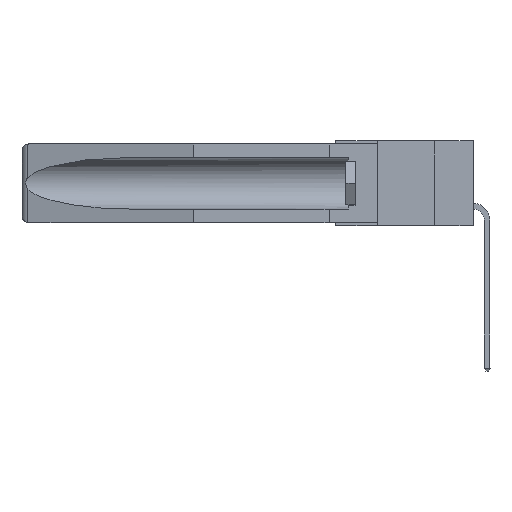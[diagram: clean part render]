
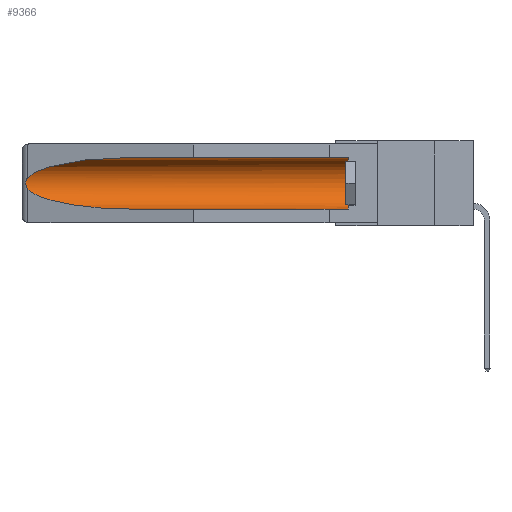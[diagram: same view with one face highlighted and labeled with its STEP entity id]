
A CAD part, left-side view. The second image highlights one B-rep face of the part: STEP entity #9366.
In plain terms, the highlighted cylindrical face has radius 2.857 mm (diameter 5.715 mm), a partial arc.
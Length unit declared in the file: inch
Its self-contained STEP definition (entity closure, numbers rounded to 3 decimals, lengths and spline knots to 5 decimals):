
#129 = CARTESIAN_POINT ( 'NONE',  ( 0.26654, 1.53092, -0.15636 ) ) ;
#334 = CARTESIAN_POINT ( 'NONE',  ( 0.21114, 1.30732, -0.284 ) ) ;
#395 = LINE ( 'NONE', #983, #7220 ) ;
#399 = CARTESIAN_POINT ( 'NONE',  ( 0.155, 0.126, -0.059 ) ) ;
#403 = ORIENTED_EDGE ( 'NONE', *, *, #19770, .T. ) ;
#882 = EDGE_CURVE ( 'NONE', #8892, #11822, #16762, .T. ) ;
#983 = CARTESIAN_POINT ( 'NONE',  ( 0.155, -0.30754, -0.059 ) ) ;
#1726 = EDGE_CURVE ( 'NONE', #2985, #11822, #15769, .T. ) ;
#1744 = CARTESIAN_POINT ( 'NONE',  ( 0.2673, 1.53269, -0.17917 ) ) ;
#1752 = CARTESIAN_POINT ( 'NONE',  ( 0.25451, 1.48313, -0.09465 ) ) ;
#2117 = CARTESIAN_POINT ( 'NONE',  ( 0.26537, 1.52718, -0.19328 ) ) ;
#2985 = VERTEX_POINT ( 'NONE', #2117 ) ;
#3013 = ORIENTED_EDGE ( 'NONE', *, *, #8179, .T. ) ;
#3300 = AXIS2_PLACEMENT_3D ( 'NONE', #17911, #8247, #13104 ) ;
#3367 = CARTESIAN_POINT ( 'NONE',  ( 0.26537, 1.52718, -0.19328 ) ) ;
#3433 = CARTESIAN_POINT ( 'NONE',  ( 0.25451, 1.48313, -0.24835 ) ) ;
#3542 = VERTEX_POINT ( 'NONE', #399 ) ;
#4724 = CYLINDRICAL_SURFACE ( 'NONE', #6456, 0.1125 ) ;
#4879 = CARTESIAN_POINT ( 'NONE',  ( 0.26597, 1.5296, -0.19026 ) ) ;
#5089 = CARTESIAN_POINT ( 'NONE',  ( 0.155, 1.07973, -0.284 ) ) ;
#6266 = DIRECTION ( 'NONE',  ( 0., 1., 0. ) ) ;
#6456 = AXIS2_PLACEMENT_3D ( 'NONE', #15570, #17184, #18846 ) ;
#6930 = CARTESIAN_POINT ( 'NONE',  ( 0.155, 0.126, -0.284 ) ) ;
#7220 = VECTOR ( 'NONE', #8891, 39.37008 ) ;
#8179 = EDGE_CURVE ( 'NONE', #18957, #16671, #12662, .T. ) ;
#8247 = DIRECTION ( 'NONE',  ( 0., -1., 0. ) ) ;
#8891 = DIRECTION ( 'NONE',  ( 0., 1., 0. ) ) ;
#8892 = VERTEX_POINT ( 'NONE', #6930 ) ;
#9040 = CARTESIAN_POINT ( 'NONE',  ( 0.155, 1.07973, -0.059 ) ) ;
#9366 = ADVANCED_FACE ( 'NONE', ( #10301 ), #4724, .F. ) ;
#9506 = CARTESIAN_POINT ( 'NONE',  ( 0.26537, 1.52718, -0.14972 ) ) ;
#9737 = CARTESIAN_POINT ( 'NONE',  ( 0.155, 1.07973, -0.059 ) ) ;
#9948 = CARTESIAN_POINT ( 'NONE',  ( 0.2675, 1.53308, -0.17534 ) ) ;
#10095 = CARTESIAN_POINT ( 'NONE',  ( 0.26537, 1.52718, -0.14972 ) ) ;
#10301 = FACE_OUTER_BOUND ( 'NONE', #13452, .T. ) ;
#11099 = B_SPLINE_CURVE_WITH_KNOTS ( 'NONE', 3,
 ( #13170, #17970, #129, #14580, #14729, #9948, #1744, #13092, #4879, #16189 ),
 .UNSPECIFIED., .F., .F.,
 ( 4, 2, 2, 2, 4 ),
 ( 0., 0.00029, 0.00058, 0.00087, 0.00117 ),
 .UNSPECIFIED. ) ;
#11822 = VERTEX_POINT ( 'NONE', #19380 ) ;
#11911 = ORIENTED_EDGE ( 'NONE', *, *, #18937, .T. ) ;
#12368 = CIRCLE ( 'NONE', #3300, 0.1125 ) ;
#12662 =( BOUNDED_CURVE ( )  B_SPLINE_CURVE ( 3, ( #9737, #12726, #1752, #10095 ),
 .UNSPECIFIED., .F., .F. ) 
 B_SPLINE_CURVE_WITH_KNOTS ( ( 4, 4 ),
 ( 4.71239, 6.08839 ),
 .UNSPECIFIED. ) 
 CURVE ( )  GEOMETRIC_REPRESENTATION_ITEM ( )  RATIONAL_B_SPLINE_CURVE ( ( 1., 0.848, 0.848, 1. ) ) 
 REPRESENTATION_ITEM ( '' )  );
#12726 = CARTESIAN_POINT ( 'NONE',  ( 0.21114, 1.30732, -0.059 ) ) ;
#13092 = CARTESIAN_POINT ( 'NONE',  ( 0.26655, 1.53094, -0.18657 ) ) ;
#13104 = DIRECTION ( 'NONE',  ( 0., 0., 1. ) ) ;
#13170 = CARTESIAN_POINT ( 'NONE',  ( 0.26537, 1.52718, -0.14972 ) ) ;
#13452 = EDGE_LOOP ( 'NONE', ( #3013, #403, #13462, #18812, #20100, #11911 ) ) ;
#13462 = ORIENTED_EDGE ( 'NONE', *, *, #1726, .T. ) ;
#14580 = CARTESIAN_POINT ( 'NONE',  ( 0.2673, 1.5327, -0.16383 ) ) ;
#14729 = CARTESIAN_POINT ( 'NONE',  ( 0.2675, 1.53308, -0.16763 ) ) ;
#15543 = EDGE_CURVE ( 'NONE', #8892, #3542, #12368, .T. ) ;
#15570 = CARTESIAN_POINT ( 'NONE',  ( 0.155, -0.30754, -0.1715 ) ) ;
#15769 =( BOUNDED_CURVE ( )  B_SPLINE_CURVE ( 3, ( #3367, #3433, #334, #5089 ),
 .UNSPECIFIED., .F., .T. ) 
 B_SPLINE_CURVE_WITH_KNOTS ( ( 4, 4 ),
 ( 0.1948, 1.5708 ),
 .UNSPECIFIED. ) 
 CURVE ( )  GEOMETRIC_REPRESENTATION_ITEM ( )  RATIONAL_B_SPLINE_CURVE ( ( 1., 0.848, 0.848, 1. ) ) 
 REPRESENTATION_ITEM ( '' )  );
#16189 = CARTESIAN_POINT ( 'NONE',  ( 0.26537, 1.52718, -0.19328 ) ) ;
#16671 = VERTEX_POINT ( 'NONE', #9506 ) ;
#16762 = LINE ( 'NONE', #19257, #20065 ) ;
#17184 = DIRECTION ( 'NONE',  ( 0., 1., 0. ) ) ;
#17911 = CARTESIAN_POINT ( 'NONE',  ( 0.155, 0.126, -0.1715 ) ) ;
#17970 = CARTESIAN_POINT ( 'NONE',  ( 0.26597, 1.52961, -0.15275 ) ) ;
#18812 = ORIENTED_EDGE ( 'NONE', *, *, #882, .F. ) ;
#18846 = DIRECTION ( 'NONE',  ( 0., 0., 1. ) ) ;
#18937 = EDGE_CURVE ( 'NONE', #3542, #18957, #395, .T. ) ;
#18957 = VERTEX_POINT ( 'NONE', #9040 ) ;
#19257 = CARTESIAN_POINT ( 'NONE',  ( 0.155, -0.30754, -0.284 ) ) ;
#19380 = CARTESIAN_POINT ( 'NONE',  ( 0.155, 1.07973, -0.284 ) ) ;
#19770 = EDGE_CURVE ( 'NONE', #16671, #2985, #11099, .T. ) ;
#20065 = VECTOR ( 'NONE', #6266, 39.37008 ) ;
#20100 = ORIENTED_EDGE ( 'NONE', *, *, #15543, .T. ) ;
